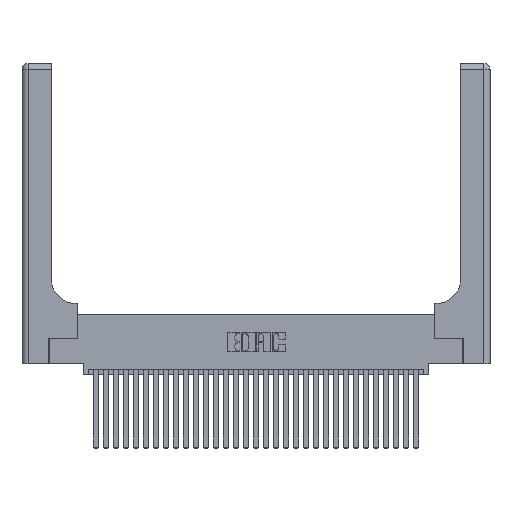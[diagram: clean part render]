
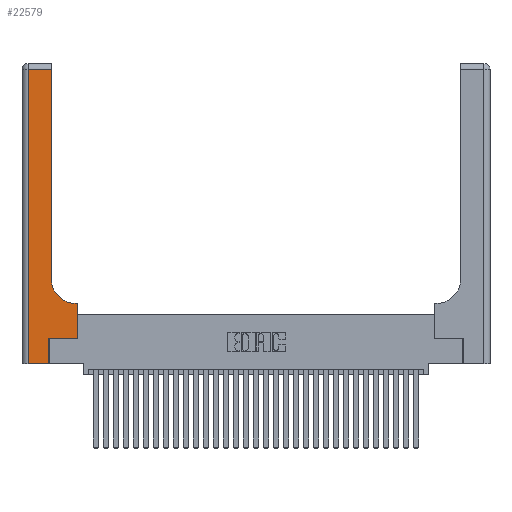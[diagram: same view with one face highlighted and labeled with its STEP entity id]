
A CAD part, top view. The second image highlights one B-rep face of the part: STEP entity #22579.
In plain terms, the highlighted planar face has unit normal (0, 0, 1).
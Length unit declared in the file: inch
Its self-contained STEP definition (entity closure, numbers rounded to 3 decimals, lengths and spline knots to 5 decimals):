
#253 = VERTEX_POINT ( 'NONE', #4450 ) ;
#837 = DIRECTION ( 'NONE',  ( 0., 1., 0. ) ) ;
#865 = VECTOR ( 'NONE', #1945, 39.37008 ) ;
#870 = VERTEX_POINT ( 'NONE', #12257 ) ;
#1150 = DIRECTION ( 'NONE',  ( 0., 1., 0. ) ) ;
#1393 = ORIENTED_EDGE ( 'NONE', *, *, #29887, .T. ) ;
#1927 = CARTESIAN_POINT ( 'NONE',  ( 0.2915, 0.6, 0.37 ) ) ;
#1945 = DIRECTION ( 'NONE',  ( 1., 0., 0. ) ) ;
#2481 = VECTOR ( 'NONE', #16822, 39.37008 ) ;
#3323 = DIRECTION ( 'NONE',  ( 0., -1., 0. ) ) ;
#3536 = EDGE_CURVE ( 'NONE', #6048, #18032, #7200, .T. ) ;
#3607 = CARTESIAN_POINT ( 'NONE',  ( 0., 0., 0.37 ) ) ;
#3865 = DIRECTION ( 'NONE',  ( 0., 0., -1. ) ) ;
#4266 = VERTEX_POINT ( 'NONE', #11458 ) ;
#4337 = CARTESIAN_POINT ( 'NONE',  ( 0., 2.94, 0.37 ) ) ;
#4450 = CARTESIAN_POINT ( 'NONE',  ( 0.269, 0.25, 0.37 ) ) ;
#5417 = LINE ( 'NONE', #4337, #12853 ) ;
#5816 = CARTESIAN_POINT ( 'NONE',  ( 0.06, 3., 0.37 ) ) ;
#6048 = VERTEX_POINT ( 'NONE', #20679 ) ;
#6107 = DIRECTION ( 'NONE',  ( 1., 0., 0. ) ) ;
#6741 = PLANE ( 'NONE',  #10282 ) ;
#6765 = LINE ( 'NONE', #31731, #865 ) ;
#6918 = ORIENTED_EDGE ( 'NONE', *, *, #23064, .T. ) ;
#7200 = LINE ( 'NONE', #5816, #32039 ) ;
#7644 = LINE ( 'NONE', #3607, #30906 ) ;
#8072 = ORIENTED_EDGE ( 'NONE', *, *, #32149, .T. ) ;
#8472 = CARTESIAN_POINT ( 'NONE',  ( 0.5585, 0.6, 0.37 ) ) ;
#8566 = VECTOR ( 'NONE', #837, 39.37008 ) ;
#8814 = ORIENTED_EDGE ( 'NONE', *, *, #3536, .T. ) ;
#9230 = DIRECTION ( 'NONE',  ( -1., 0., 0. ) ) ;
#9825 = CARTESIAN_POINT ( 'NONE',  ( 0.269, 0., 0.37 ) ) ;
#10282 = AXIS2_PLACEMENT_3D ( 'NONE', #31471, #24053, #9230 ) ;
#10756 = ORIENTED_EDGE ( 'NONE', *, *, #12919, .T. ) ;
#11458 = CARTESIAN_POINT ( 'NONE',  ( 0.2915, 0.85, 0.37 ) ) ;
#11535 = VERTEX_POINT ( 'NONE', #15643 ) ;
#11713 = CARTESIAN_POINT ( 'NONE',  ( 0.5585, 0.25, 0.37 ) ) ;
#12257 = CARTESIAN_POINT ( 'NONE',  ( 0.2915, 2.94, 0.37 ) ) ;
#12463 = VECTOR ( 'NONE', #29325, 39.37008 ) ;
#12853 = VECTOR ( 'NONE', #21664, 39.37008 ) ;
#12877 = LINE ( 'NONE', #13608, #18635 ) ;
#12919 = EDGE_CURVE ( 'NONE', #870, #6048, #5417, .T. ) ;
#13608 = CARTESIAN_POINT ( 'NONE',  ( 0.2915, 3., 0.37 ) ) ;
#14547 = FACE_OUTER_BOUND ( 'NONE', #17161, .T. ) ;
#14659 = VERTEX_POINT ( 'NONE', #11713 ) ;
#15447 = ORIENTED_EDGE ( 'NONE', *, *, #25763, .T. ) ;
#15479 = ORIENTED_EDGE ( 'NONE', *, *, #26601, .T. ) ;
#15643 = CARTESIAN_POINT ( 'NONE',  ( 0.5415, 0.6, 0.37 ) ) ;
#16822 = DIRECTION ( 'NONE',  ( 0., 1., 0. ) ) ;
#17007 = ORIENTED_EDGE ( 'NONE', *, *, #30214, .T. ) ;
#17161 = EDGE_LOOP ( 'NONE', ( #22335, #10756, #8814, #15447, #1393, #8072, #15479, #17007, #6918 ) ) ;
#17372 = CARTESIAN_POINT ( 'NONE',  ( 0.06, 0., 0.37 ) ) ;
#18032 = VERTEX_POINT ( 'NONE', #17372 ) ;
#18635 = VECTOR ( 'NONE', #1150, 39.37008 ) ;
#18725 = CARTESIAN_POINT ( 'NONE',  ( 0.5415, 0.85, 0.37 ) ) ;
#20679 = CARTESIAN_POINT ( 'NONE',  ( 0.06, 2.94, 0.37 ) ) ;
#21180 = DIRECTION ( 'NONE',  ( 1., 0., 0. ) ) ;
#21664 = DIRECTION ( 'NONE',  ( -1., 0., 0. ) ) ;
#21723 = LINE ( 'NONE', #30631, #8566 ) ;
#22335 = ORIENTED_EDGE ( 'NONE', *, *, #29977, .T. ) ;
#22579 = ADVANCED_FACE ( 'NONE', ( #14547 ), #6741, .F. ) ;
#22883 = AXIS2_PLACEMENT_3D ( 'NONE', #18725, #3865, #21180 ) ;
#23064 = EDGE_CURVE ( 'NONE', #11535, #4266, #27695, .T. ) ;
#24053 = DIRECTION ( 'NONE',  ( 0., 0., -1. ) ) ;
#25151 = VERTEX_POINT ( 'NONE', #9825 ) ;
#25763 = EDGE_CURVE ( 'NONE', #18032, #25151, #7644, .T. ) ;
#26355 = VERTEX_POINT ( 'NONE', #8472 ) ;
#26601 = EDGE_CURVE ( 'NONE', #14659, #26355, #27375, .T. ) ;
#27375 = LINE ( 'NONE', #31680, #2481 ) ;
#27695 = CIRCLE ( 'NONE', #22883, 0.25 ) ;
#29325 = DIRECTION ( 'NONE',  ( -1., 0., 0. ) ) ;
#29887 = EDGE_CURVE ( 'NONE', #25151, #253, #21723, .T. ) ;
#29977 = EDGE_CURVE ( 'NONE', #4266, #870, #12877, .T. ) ;
#30214 = EDGE_CURVE ( 'NONE', #26355, #11535, #32262, .T. ) ;
#30631 = CARTESIAN_POINT ( 'NONE',  ( 0.269, 0., 0.37 ) ) ;
#30906 = VECTOR ( 'NONE', #6107, 39.37008 ) ;
#31471 = CARTESIAN_POINT ( 'NONE',  ( 0., 3., 0.37 ) ) ;
#31680 = CARTESIAN_POINT ( 'NONE',  ( 0.5585, 0.25, 0.37 ) ) ;
#31731 = CARTESIAN_POINT ( 'NONE',  ( 0.269, 0.25, 0.37 ) ) ;
#32039 = VECTOR ( 'NONE', #3323, 39.37008 ) ;
#32149 = EDGE_CURVE ( 'NONE', #253, #14659, #6765, .T. ) ;
#32262 = LINE ( 'NONE', #1927, #12463 ) ;
